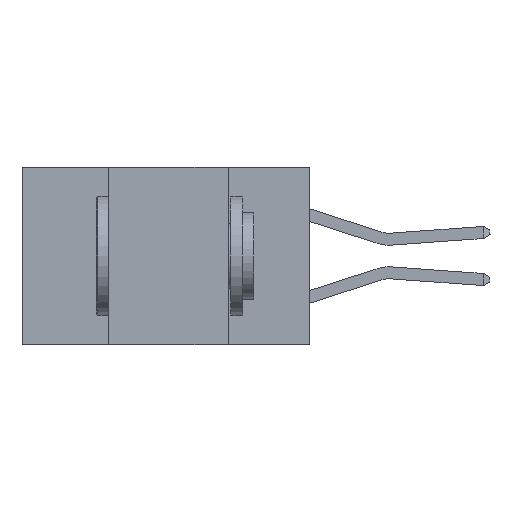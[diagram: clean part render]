
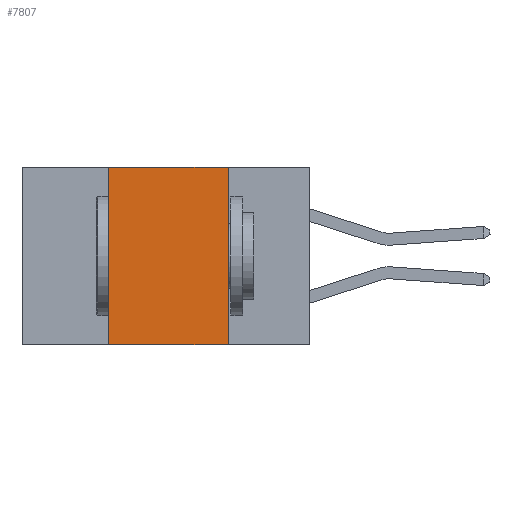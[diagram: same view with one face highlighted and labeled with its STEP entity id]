
A CAD part, left-side view. The second image highlights one B-rep face of the part: STEP entity #7807.
In plain terms, the highlighted planar face has unit normal (-1, 0, 0).
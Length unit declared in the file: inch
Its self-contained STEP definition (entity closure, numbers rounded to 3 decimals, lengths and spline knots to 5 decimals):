
#370 = LINE ( 'NONE', #13558, #6925 ) ;
#616 = CARTESIAN_POINT ( 'NONE',  ( 0., 0.17, -0.37 ) ) ;
#756 = CARTESIAN_POINT ( 'NONE',  ( 0., 0.42, 0. ) ) ;
#1825 = EDGE_CURVE ( 'NONE', #8007, #10847, #370, .T. ) ;
#3816 = CARTESIAN_POINT ( 'NONE',  ( 0., 0.6, 0. ) ) ;
#4639 = ORIENTED_EDGE ( 'NONE', *, *, #21687, .F. ) ;
#4666 = PLANE ( 'NONE',  #20756 ) ;
#4827 = CARTESIAN_POINT ( 'NONE',  ( 0., 0.6, -0.37 ) ) ;
#4916 = LINE ( 'NONE', #11791, #8667 ) ;
#5054 = DIRECTION ( 'NONE',  ( 0., -1., 0. ) ) ;
#6859 = LINE ( 'NONE', #4827, #15135 ) ;
#6925 = VECTOR ( 'NONE', #15501, 39.37008 ) ;
#6978 = LINE ( 'NONE', #3816, #15523 ) ;
#7708 = VERTEX_POINT ( 'NONE', #756 ) ;
#7807 = ADVANCED_FACE ( 'NONE', ( #18433 ), #4666, .F. ) ;
#8007 = VERTEX_POINT ( 'NONE', #16959 ) ;
#8667 = VECTOR ( 'NONE', #20154, 39.37008 ) ;
#10847 = VERTEX_POINT ( 'NONE', #616 ) ;
#11789 = CARTESIAN_POINT ( 'NONE',  ( 0., 0.42, -0.37 ) ) ;
#11791 = CARTESIAN_POINT ( 'NONE',  ( 0., 0.42, -0.37 ) ) ;
#12114 = EDGE_LOOP ( 'NONE', ( #19753, #14896, #4639, #17684 ) ) ;
#13240 = EDGE_CURVE ( 'NONE', #18732, #10847, #6859, .T. ) ;
#13558 = CARTESIAN_POINT ( 'NONE',  ( 0., 0.17, -0.37 ) ) ;
#14610 = DIRECTION ( 'NONE',  ( 0., 0., -1. ) ) ;
#14896 = ORIENTED_EDGE ( 'NONE', *, *, #21289, .F. ) ;
#14934 = CARTESIAN_POINT ( 'NONE',  ( 0., 0.6, 0. ) ) ;
#15045 = DIRECTION ( 'NONE',  ( 1., 0., 0. ) ) ;
#15135 = VECTOR ( 'NONE', #5054, 39.37008 ) ;
#15501 = DIRECTION ( 'NONE',  ( 0., 0., -1. ) ) ;
#15523 = VECTOR ( 'NONE', #17581, 39.37008 ) ;
#16959 = CARTESIAN_POINT ( 'NONE',  ( 0., 0.17, 0. ) ) ;
#17581 = DIRECTION ( 'NONE',  ( 0., -1., 0. ) ) ;
#17684 = ORIENTED_EDGE ( 'NONE', *, *, #13240, .T. ) ;
#18433 = FACE_OUTER_BOUND ( 'NONE', #12114, .T. ) ;
#18732 = VERTEX_POINT ( 'NONE', #11789 ) ;
#19753 = ORIENTED_EDGE ( 'NONE', *, *, #1825, .F. ) ;
#20154 = DIRECTION ( 'NONE',  ( 0., 0., 1. ) ) ;
#20756 = AXIS2_PLACEMENT_3D ( 'NONE', #14934, #15045, #14610 ) ;
#21289 = EDGE_CURVE ( 'NONE', #7708, #8007, #6978, .T. ) ;
#21687 = EDGE_CURVE ( 'NONE', #18732, #7708, #4916, .T. ) ;
